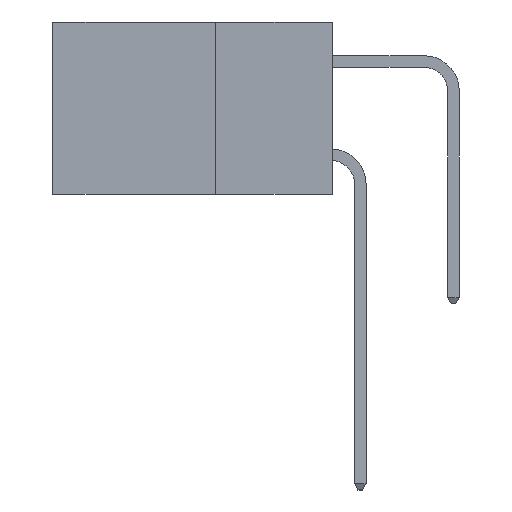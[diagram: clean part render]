
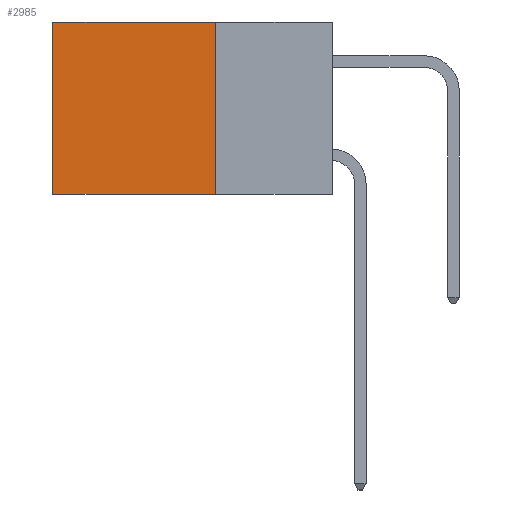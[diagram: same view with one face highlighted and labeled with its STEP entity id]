
A CAD part, left-side view. The second image highlights one B-rep face of the part: STEP entity #2985.
In plain terms, the highlighted planar face has unit normal (-1, 0, 0).
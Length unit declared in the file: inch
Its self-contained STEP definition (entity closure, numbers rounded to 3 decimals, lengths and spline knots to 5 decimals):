
#767 = CARTESIAN_POINT ( 'NONE',  ( 0.2615, 0.6, -0.37 ) ) ;
#1049 = VECTOR ( 'NONE', #5518, 39.37008 ) ;
#1854 = VECTOR ( 'NONE', #14126, 39.37008 ) ;
#2160 = AXIS2_PLACEMENT_3D ( 'NONE', #8670, #8491, #8307 ) ;
#2654 = DIRECTION ( 'NONE',  ( 0., 0., -1. ) ) ;
#2985 = ADVANCED_FACE ( 'NONE', ( #13555 ), #8741, .F. ) ;
#3996 = EDGE_CURVE ( 'NONE', #7798, #11690, #13381, .T. ) ;
#4351 = CARTESIAN_POINT ( 'NONE',  ( 0.2615, 0.25, -0.37 ) ) ;
#4834 = ORIENTED_EDGE ( 'NONE', *, *, #14134, .F. ) ;
#5315 = VECTOR ( 'NONE', #12376, 39.37008 ) ;
#5485 = VERTEX_POINT ( 'NONE', #13996 ) ;
#5518 = DIRECTION ( 'NONE',  ( 0., 0., -1. ) ) ;
#6523 = VERTEX_POINT ( 'NONE', #767 ) ;
#7719 = EDGE_CURVE ( 'NONE', #7798, #5485, #7731, .T. ) ;
#7731 = LINE ( 'NONE', #8382, #1854 ) ;
#7798 = VERTEX_POINT ( 'NONE', #9687 ) ;
#7999 = LINE ( 'NONE', #4351, #5315 ) ;
#8079 = EDGE_LOOP ( 'NONE', ( #12189, #4834, #8254, #9339 ) ) ;
#8254 = ORIENTED_EDGE ( 'NONE', *, *, #3996, .F. ) ;
#8307 = DIRECTION ( 'NONE',  ( 0., 0., -1. ) ) ;
#8382 = CARTESIAN_POINT ( 'NONE',  ( 0.2615, 0.25, 0. ) ) ;
#8491 = DIRECTION ( 'NONE',  ( 1., 0., 0. ) ) ;
#8670 = CARTESIAN_POINT ( 'NONE',  ( 0.2615, 0.25, -0.37 ) ) ;
#8741 = PLANE ( 'NONE',  #2160 ) ;
#9339 = ORIENTED_EDGE ( 'NONE', *, *, #7719, .T. ) ;
#9687 = CARTESIAN_POINT ( 'NONE',  ( 0.2615, 0.25, 0. ) ) ;
#10502 = LINE ( 'NONE', #10782, #13185 ) ;
#10782 = CARTESIAN_POINT ( 'NONE',  ( 0.2615, 0.6, -0.37 ) ) ;
#11690 = VERTEX_POINT ( 'NONE', #14649 ) ;
#12189 = ORIENTED_EDGE ( 'NONE', *, *, #14407, .T. ) ;
#12376 = DIRECTION ( 'NONE',  ( 0., 1., 0. ) ) ;
#12726 = CARTESIAN_POINT ( 'NONE',  ( 0.2615, 0.25, -0.37 ) ) ;
#13185 = VECTOR ( 'NONE', #2654, 39.37008 ) ;
#13381 = LINE ( 'NONE', #12726, #1049 ) ;
#13555 = FACE_OUTER_BOUND ( 'NONE', #8079, .T. ) ;
#13996 = CARTESIAN_POINT ( 'NONE',  ( 0.2615, 0.6, 0. ) ) ;
#14126 = DIRECTION ( 'NONE',  ( 0., 1., 0. ) ) ;
#14134 = EDGE_CURVE ( 'NONE', #11690, #6523, #7999, .T. ) ;
#14407 = EDGE_CURVE ( 'NONE', #5485, #6523, #10502, .T. ) ;
#14649 = CARTESIAN_POINT ( 'NONE',  ( 0.2615, 0.25, -0.37 ) ) ;
